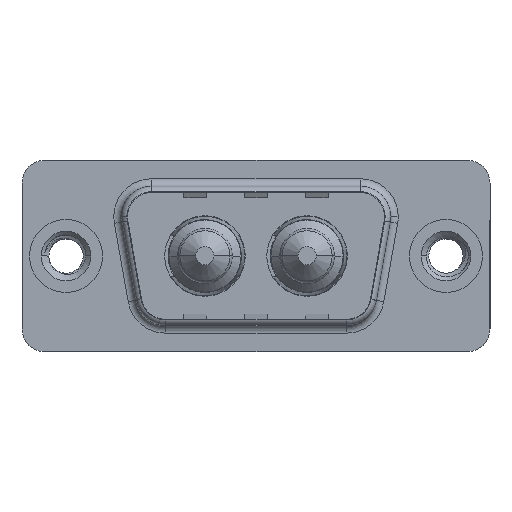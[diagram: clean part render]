
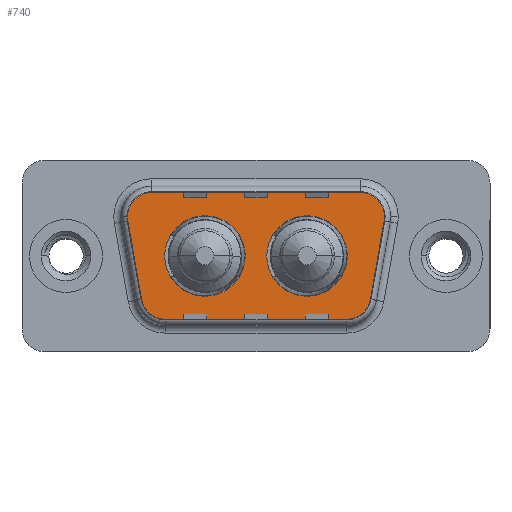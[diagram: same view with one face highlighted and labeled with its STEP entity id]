
A CAD part, top view. The second image highlights one B-rep face of the part: STEP entity #740.
In plain terms, the highlighted planar face has unit normal (0, 0, 1).
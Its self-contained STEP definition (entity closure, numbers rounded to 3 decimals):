
#67 = VERTEX_POINT ( 'NONE', #8244 ) ;
#257 = VERTEX_POINT ( 'NONE', #438 ) ;
#438 = CARTESIAN_POINT ( 'NONE',  ( 5.436, 4.9, 0. ) ) ;
#740 = ADVANCED_FACE ( 'NONE', ( #13182, #6364, #9944 ), #14653, .T. ) ;
#857 = DIRECTION ( 'NONE',  ( -1., 0., 0. ) ) ;
#892 = AXIS2_PLACEMENT_3D ( 'NONE', #2072, #10566, #3307 ) ;
#923 = DIRECTION ( 'NONE',  ( -1., 0., 0. ) ) ;
#954 = DIRECTION ( 'NONE',  ( 0., 0., 1. ) ) ;
#990 = LINE ( 'NONE', #8513, #10718 ) ;
#1111 = AXIS2_PLACEMENT_3D ( 'NONE', #1665, #10187, #2918 ) ;
#1347 = LINE ( 'NONE', #11910, #7501 ) ;
#1497 = EDGE_CURVE ( 'NONE', #257, #3802, #5232, .T. ) ;
#1573 = AXIS2_PLACEMENT_3D ( 'NONE', #15009, #13722, #1937 ) ;
#1654 = CARTESIAN_POINT ( 'NONE',  ( 21.564, 2.9, 0. ) ) ;
#1665 = CARTESIAN_POINT ( 'NONE',  ( 18.541, -2.9, 0. ) ) ;
#1748 = ORIENTED_EDGE ( 'NONE', *, *, #4825, .T. ) ;
#1754 = CARTESIAN_POINT ( 'NONE',  ( 3.466, 2.553, 0. ) ) ;
#1856 = DIRECTION ( 'NONE',  ( 1., 0., 0. ) ) ;
#1937 = DIRECTION ( 'NONE',  ( 1., 0., 0. ) ) ;
#1954 = DIRECTION ( 'NONE',  ( 0., 0., 1. ) ) ;
#2007 = ORIENTED_EDGE ( 'NONE', *, *, #13575, .F. ) ;
#2058 = DIRECTION ( 'NONE',  ( 0., 0., 1. ) ) ;
#2070 = ORIENTED_EDGE ( 'NONE', *, *, #6331, .T. ) ;
#2072 = CARTESIAN_POINT ( 'NONE',  ( 19.564, 2.9, 0. ) ) ;
#2220 = EDGE_LOOP ( 'NONE', ( #2007, #9641 ) ) ;
#2345 = AXIS2_PLACEMENT_3D ( 'NONE', #12245, #5023, #13481 ) ;
#2419 = VERTEX_POINT ( 'NONE', #8393 ) ;
#2493 = CIRCLE ( 'NONE', #15054, 2.65 ) ;
#2519 = CARTESIAN_POINT ( 'NONE',  ( 3.466, 2.553, 0. ) ) ;
#2628 = CIRCLE ( 'NONE', #6841, 2.65 ) ;
#2918 = DIRECTION ( 'NONE',  ( 1., 0., 0. ) ) ;
#2921 = ORIENTED_EDGE ( 'NONE', *, *, #11826, .T. ) ;
#3014 = DIRECTION ( 'NONE',  ( 0.174, -0.985, 0. ) ) ;
#3307 = DIRECTION ( 'NONE',  ( -1., 0., 0. ) ) ;
#3488 = LINE ( 'NONE', #13056, #15624 ) ;
#3802 = VERTEX_POINT ( 'NONE', #2519 ) ;
#3837 = EDGE_LOOP ( 'NONE', ( #15372, #4381, #10563, #9951, #5068, #10400, #2070, #2921, #1748 ) ) ;
#3903 = VERTEX_POINT ( 'NONE', #13401 ) ;
#4381 = ORIENTED_EDGE ( 'NONE', *, *, #8427, .T. ) ;
#4607 = CARTESIAN_POINT ( 'NONE',  ( 4.489, -3.247, 0. ) ) ;
#4612 = CIRCLE ( 'NONE', #892, 2. ) ;
#4825 = EDGE_CURVE ( 'NONE', #12643, #67, #1347, .T. ) ;
#5023 = DIRECTION ( 'NONE',  ( 0., 0., 1. ) ) ;
#5068 = ORIENTED_EDGE ( 'NONE', *, *, #7848, .T. ) ;
#5232 = CIRCLE ( 'NONE', #1573, 2. ) ;
#5255 = CIRCLE ( 'NONE', #1111, 2. ) ;
#5810 = DIRECTION ( 'NONE',  ( 0.174, 0.985, 0. ) ) ;
#5867 = EDGE_CURVE ( 'NONE', #14993, #9448, #7288, .T. ) ;
#5894 = VERTEX_POINT ( 'NONE', #4607 ) ;
#5902 = DIRECTION ( 'NONE',  ( 1., 0., 0. ) ) ;
#6073 = EDGE_CURVE ( 'NONE', #7228, #2419, #11047, .T. ) ;
#6146 = AXIS2_PLACEMENT_3D ( 'NONE', #6620, #15074, #7858 ) ;
#6331 = EDGE_CURVE ( 'NONE', #3802, #5894, #9154, .T. ) ;
#6364 = FACE_BOUND ( 'NONE', #2220, .T. ) ;
#6620 = CARTESIAN_POINT ( 'NONE',  ( 15.86, 0., 0. ) ) ;
#6633 = EDGE_CURVE ( 'NONE', #2419, #7228, #6885, .T. ) ;
#6770 = EDGE_CURVE ( 'NONE', #10742, #10035, #2493, .T. ) ;
#6841 = AXIS2_PLACEMENT_3D ( 'NONE', #8285, #954, #9502 ) ;
#6847 = EDGE_CURVE ( 'NONE', #9448, #3903, #4612, .T. ) ;
#6885 = CIRCLE ( 'NONE', #6146, 2.65 ) ;
#7186 = CARTESIAN_POINT ( 'NONE',  ( 21.534, 2.553, 0. ) ) ;
#7228 = VERTEX_POINT ( 'NONE', #12416 ) ;
#7288 = CIRCLE ( 'NONE', #7559, 2. ) ;
#7333 = EDGE_CURVE ( 'NONE', #67, #10156, #5255, .T. ) ;
#7501 = VECTOR ( 'NONE', #5902, 1000. ) ;
#7559 = AXIS2_PLACEMENT_3D ( 'NONE', #15483, #8247, #923 ) ;
#7636 = ORIENTED_EDGE ( 'NONE', *, *, #6073, .F. ) ;
#7698 = CARTESIAN_POINT ( 'NONE',  ( 11.79, 0., 0. ) ) ;
#7848 = EDGE_CURVE ( 'NONE', #3903, #257, #990, .T. ) ;
#7858 = DIRECTION ( 'NONE',  ( 1., 0., 0. ) ) ;
#8145 = CARTESIAN_POINT ( 'NONE',  ( 18.541, -2.9, 0. ) ) ;
#8194 = DIRECTION ( 'NONE',  ( 0., 0., 1. ) ) ;
#8244 = CARTESIAN_POINT ( 'NONE',  ( 18.541, -4.9, 0. ) ) ;
#8247 = DIRECTION ( 'NONE',  ( 0., 0., 1. ) ) ;
#8285 = CARTESIAN_POINT ( 'NONE',  ( 9.14, 0., 0. ) ) ;
#8393 = CARTESIAN_POINT ( 'NONE',  ( 13.21, 0., 0. ) ) ;
#8427 = EDGE_CURVE ( 'NONE', #10156, #14993, #3488, .T. ) ;
#8513 = CARTESIAN_POINT ( 'NONE',  ( 5.436, 4.9, 0. ) ) ;
#9154 = LINE ( 'NONE', #1754, #15209 ) ;
#9256 = CARTESIAN_POINT ( 'NONE',  ( 9.14, 0., 0. ) ) ;
#9265 = EDGE_LOOP ( 'NONE', ( #7636, #13459 ) ) ;
#9448 = VERTEX_POINT ( 'NONE', #1654 ) ;
#9502 = DIRECTION ( 'NONE',  ( 1., 0., 0. ) ) ;
#9641 = ORIENTED_EDGE ( 'NONE', *, *, #6770, .F. ) ;
#9845 = AXIS2_PLACEMENT_3D ( 'NONE', #8145, #2058, #1856 ) ;
#9944 = FACE_OUTER_BOUND ( 'NONE', #3837, .T. ) ;
#9951 = ORIENTED_EDGE ( 'NONE', *, *, #6847, .T. ) ;
#10035 = VERTEX_POINT ( 'NONE', #7698 ) ;
#10156 = VERTEX_POINT ( 'NONE', #10731 ) ;
#10187 = DIRECTION ( 'NONE',  ( 0., 0., 1. ) ) ;
#10400 = ORIENTED_EDGE ( 'NONE', *, *, #1497, .T. ) ;
#10465 = DIRECTION ( 'NONE',  ( 1., 0., 0. ) ) ;
#10563 = ORIENTED_EDGE ( 'NONE', *, *, #5867, .T. ) ;
#10566 = DIRECTION ( 'NONE',  ( 0., 0., 1. ) ) ;
#10718 = VECTOR ( 'NONE', #14544, 1000. ) ;
#10731 = CARTESIAN_POINT ( 'NONE',  ( 20.511, -3.247, 0. ) ) ;
#10742 = VERTEX_POINT ( 'NONE', #13521 ) ;
#11047 = CIRCLE ( 'NONE', #2345, 2.65 ) ;
#11826 = EDGE_CURVE ( 'NONE', #5894, #12643, #14067, .T. ) ;
#11910 = CARTESIAN_POINT ( 'NONE',  ( 6.459, -4.9, 0. ) ) ;
#12010 = CARTESIAN_POINT ( 'NONE',  ( 6.459, -4.9, 0. ) ) ;
#12245 = CARTESIAN_POINT ( 'NONE',  ( 15.86, 0., 0. ) ) ;
#12416 = CARTESIAN_POINT ( 'NONE',  ( 18.51, 0., 0. ) ) ;
#12643 = VERTEX_POINT ( 'NONE', #12010 ) ;
#13056 = CARTESIAN_POINT ( 'NONE',  ( 21.534, 2.553, 0. ) ) ;
#13182 = FACE_BOUND ( 'NONE', #9265, .T. ) ;
#13401 = CARTESIAN_POINT ( 'NONE',  ( 19.564, 4.9, 0. ) ) ;
#13459 = ORIENTED_EDGE ( 'NONE', *, *, #6633, .F. ) ;
#13481 = DIRECTION ( 'NONE',  ( 1., 0., 0. ) ) ;
#13512 = AXIS2_PLACEMENT_3D ( 'NONE', #15429, #8194, #857 ) ;
#13521 = CARTESIAN_POINT ( 'NONE',  ( 6.49, 0., 0. ) ) ;
#13575 = EDGE_CURVE ( 'NONE', #10035, #10742, #2628, .T. ) ;
#13722 = DIRECTION ( 'NONE',  ( 0., 0., 1. ) ) ;
#14067 = CIRCLE ( 'NONE', #13512, 2. ) ;
#14544 = DIRECTION ( 'NONE',  ( -1., 0., 0. ) ) ;
#14653 = PLANE ( 'NONE',  #9845 ) ;
#14993 = VERTEX_POINT ( 'NONE', #7186 ) ;
#15009 = CARTESIAN_POINT ( 'NONE',  ( 5.436, 2.9, 0. ) ) ;
#15054 = AXIS2_PLACEMENT_3D ( 'NONE', #9256, #1954, #10465 ) ;
#15074 = DIRECTION ( 'NONE',  ( 0., 0., 1. ) ) ;
#15209 = VECTOR ( 'NONE', #3014, 1000. ) ;
#15372 = ORIENTED_EDGE ( 'NONE', *, *, #7333, .T. ) ;
#15429 = CARTESIAN_POINT ( 'NONE',  ( 6.459, -2.9, 0. ) ) ;
#15483 = CARTESIAN_POINT ( 'NONE',  ( 19.564, 2.9, 0. ) ) ;
#15624 = VECTOR ( 'NONE', #5810, 1000. ) ;
